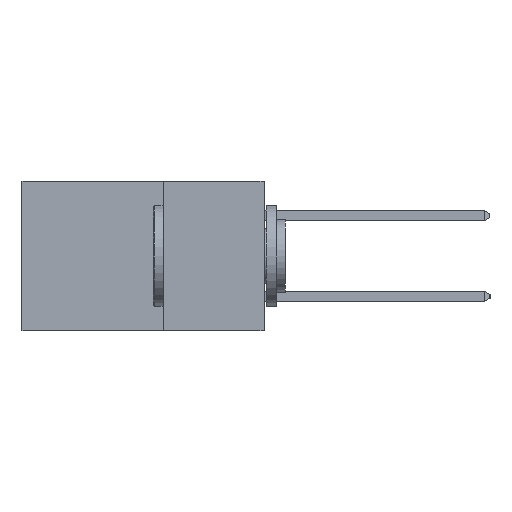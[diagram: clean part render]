
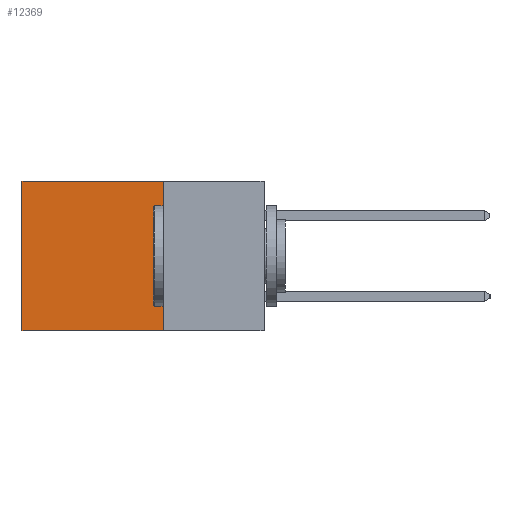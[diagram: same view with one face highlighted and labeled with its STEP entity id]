
A CAD part, left-side view. The second image highlights one B-rep face of the part: STEP entity #12369.
In plain terms, the highlighted planar face has unit normal (-1, 0, 0).
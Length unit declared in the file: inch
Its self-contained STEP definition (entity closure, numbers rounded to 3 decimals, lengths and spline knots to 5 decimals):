
#40 = DIRECTION ( 'NONE',  ( 0., 1., 0. ) ) ;
#586 = EDGE_LOOP ( 'NONE', ( #8175, #7443, #14625, #1010 ) ) ;
#1010 = ORIENTED_EDGE ( 'NONE', *, *, #20176, .T. ) ;
#1303 = AXIS2_PLACEMENT_3D ( 'NONE', #9898, #17942, #8279 ) ;
#1898 = EDGE_CURVE ( 'NONE', #17659, #3797, #7962, .T. ) ;
#1966 = LINE ( 'NONE', #9365, #2490 ) ;
#2490 = VECTOR ( 'NONE', #20454, 39.37008 ) ;
#3698 = LINE ( 'NONE', #20962, #12039 ) ;
#3797 = VERTEX_POINT ( 'NONE', #17532 ) ;
#4926 = PLANE ( 'NONE',  #1303 ) ;
#6098 = VERTEX_POINT ( 'NONE', #10180 ) ;
#7443 = ORIENTED_EDGE ( 'NONE', *, *, #19827, .F. ) ;
#7447 = VECTOR ( 'NONE', #18378, 39.37008 ) ;
#7962 = LINE ( 'NONE', #12101, #7447 ) ;
#8175 = ORIENTED_EDGE ( 'NONE', *, *, #9159, .T. ) ;
#8279 = DIRECTION ( 'NONE',  ( 0., 0., -1. ) ) ;
#8425 = CARTESIAN_POINT ( 'NONE',  ( 0.2615, 0.25, -0.37 ) ) ;
#9159 = EDGE_CURVE ( 'NONE', #20902, #6098, #3698, .T. ) ;
#9365 = CARTESIAN_POINT ( 'NONE',  ( 0.2615, 0.25, 0. ) ) ;
#9898 = CARTESIAN_POINT ( 'NONE',  ( 0.2615, 0.25, -0.37 ) ) ;
#10180 = CARTESIAN_POINT ( 'NONE',  ( 0.2615, 0.6, -0.37 ) ) ;
#12039 = VECTOR ( 'NONE', #20113, 39.37008 ) ;
#12101 = CARTESIAN_POINT ( 'NONE',  ( 0.2615, 0.25, -0.37 ) ) ;
#12369 = ADVANCED_FACE ( 'NONE', ( #19855 ), #4926, .F. ) ;
#14184 = VECTOR ( 'NONE', #40, 39.37008 ) ;
#14434 = CARTESIAN_POINT ( 'NONE',  ( 0.2615, 0.25, 0. ) ) ;
#14625 = ORIENTED_EDGE ( 'NONE', *, *, #1898, .F. ) ;
#17413 = LINE ( 'NONE', #8425, #14184 ) ;
#17532 = CARTESIAN_POINT ( 'NONE',  ( 0.2615, 0.25, -0.37 ) ) ;
#17659 = VERTEX_POINT ( 'NONE', #14434 ) ;
#17942 = DIRECTION ( 'NONE',  ( 1., 0., 0. ) ) ;
#18378 = DIRECTION ( 'NONE',  ( 0., 0., -1. ) ) ;
#18620 = CARTESIAN_POINT ( 'NONE',  ( 0.2615, 0.6, 0. ) ) ;
#19827 = EDGE_CURVE ( 'NONE', #3797, #6098, #17413, .T. ) ;
#19855 = FACE_OUTER_BOUND ( 'NONE', #586, .T. ) ;
#20113 = DIRECTION ( 'NONE',  ( 0., 0., -1. ) ) ;
#20176 = EDGE_CURVE ( 'NONE', #17659, #20902, #1966, .T. ) ;
#20454 = DIRECTION ( 'NONE',  ( 0., 1., 0. ) ) ;
#20902 = VERTEX_POINT ( 'NONE', #18620 ) ;
#20962 = CARTESIAN_POINT ( 'NONE',  ( 0.2615, 0.6, -0.37 ) ) ;
